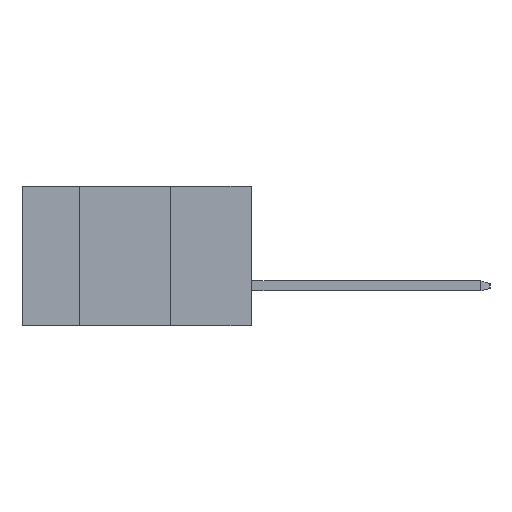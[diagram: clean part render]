
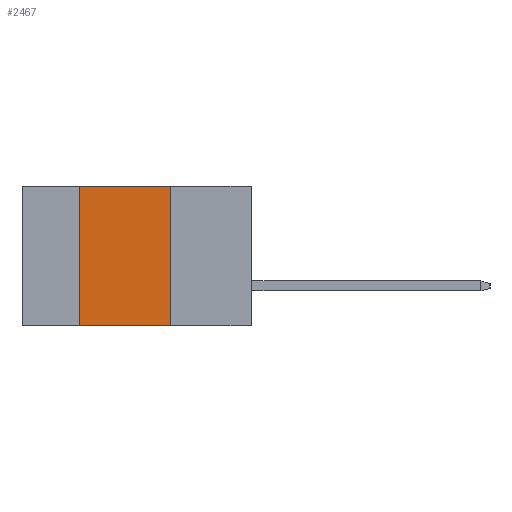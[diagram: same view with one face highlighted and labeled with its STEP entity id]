
A CAD part, left-side view. The second image highlights one B-rep face of the part: STEP entity #2467.
In plain terms, the highlighted planar face has unit normal (-1, 0, 0).
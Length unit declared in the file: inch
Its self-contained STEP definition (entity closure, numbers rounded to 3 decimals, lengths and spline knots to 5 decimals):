
#287 = CARTESIAN_POINT ( 'NONE',  ( 0., 0.72, 0. ) ) ;
#402 = CARTESIAN_POINT ( 'NONE',  ( 0., 0.254, -0.437 ) ) ;
#553 = VECTOR ( 'NONE', #4232, 39.37008 ) ;
#823 = ORIENTED_EDGE ( 'NONE', *, *, #8891, .F. ) ;
#1136 = CARTESIAN_POINT ( 'NONE',  ( 0., 0.54, 0. ) ) ;
#1725 = DIRECTION ( 'NONE',  ( 0., 0., -1. ) ) ;
#2369 = DIRECTION ( 'NONE',  ( 0., -1., 0. ) ) ;
#2467 = ADVANCED_FACE ( 'NONE', ( #5440 ), #2942, .F. ) ;
#2942 = PLANE ( 'NONE',  #8074 ) ;
#3129 = LINE ( 'NONE', #9853, #7545 ) ;
#3654 = DIRECTION ( 'NONE',  ( 0., -1., 0. ) ) ;
#4232 = DIRECTION ( 'NONE',  ( 0., 0., 1. ) ) ;
#4685 = ORIENTED_EDGE ( 'NONE', *, *, #10552, .F. ) ;
#5440 = FACE_OUTER_BOUND ( 'NONE', #10532, .T. ) ;
#5502 = DIRECTION ( 'NONE',  ( 0., 0., -1. ) ) ;
#5588 = LINE ( 'NONE', #8924, #7436 ) ;
#5595 = DIRECTION ( 'NONE',  ( 1., 0., 0. ) ) ;
#5957 = CARTESIAN_POINT ( 'NONE',  ( 0., 0.54, -0.437 ) ) ;
#5959 = VERTEX_POINT ( 'NONE', #402 ) ;
#6015 = VERTEX_POINT ( 'NONE', #10437 ) ;
#6160 = VERTEX_POINT ( 'NONE', #6474 ) ;
#6474 = CARTESIAN_POINT ( 'NONE',  ( 0., 0.54, -0.437 ) ) ;
#6787 = LINE ( 'NONE', #5957, #553 ) ;
#7436 = VECTOR ( 'NONE', #1725, 39.37008 ) ;
#7545 = VECTOR ( 'NONE', #2369, 39.37008 ) ;
#7672 = EDGE_CURVE ( 'NONE', #6015, #5959, #5588, .T. ) ;
#7797 = LINE ( 'NONE', #287, #8575 ) ;
#8004 = CARTESIAN_POINT ( 'NONE',  ( 0., 0.72, 0. ) ) ;
#8074 = AXIS2_PLACEMENT_3D ( 'NONE', #8004, #5595, #5502 ) ;
#8221 = EDGE_CURVE ( 'NONE', #6160, #5959, #3129, .T. ) ;
#8575 = VECTOR ( 'NONE', #3654, 39.37008 ) ;
#8891 = EDGE_CURVE ( 'NONE', #9187, #6015, #7797, .T. ) ;
#8924 = CARTESIAN_POINT ( 'NONE',  ( 0., 0.254, -0.437 ) ) ;
#9187 = VERTEX_POINT ( 'NONE', #1136 ) ;
#9295 = ORIENTED_EDGE ( 'NONE', *, *, #8221, .T. ) ;
#9449 = ORIENTED_EDGE ( 'NONE', *, *, #7672, .F. ) ;
#9853 = CARTESIAN_POINT ( 'NONE',  ( 0., 0.72, -0.437 ) ) ;
#10437 = CARTESIAN_POINT ( 'NONE',  ( 0., 0.254, 0. ) ) ;
#10532 = EDGE_LOOP ( 'NONE', ( #9449, #823, #4685, #9295 ) ) ;
#10552 = EDGE_CURVE ( 'NONE', #6160, #9187, #6787, .T. ) ;
